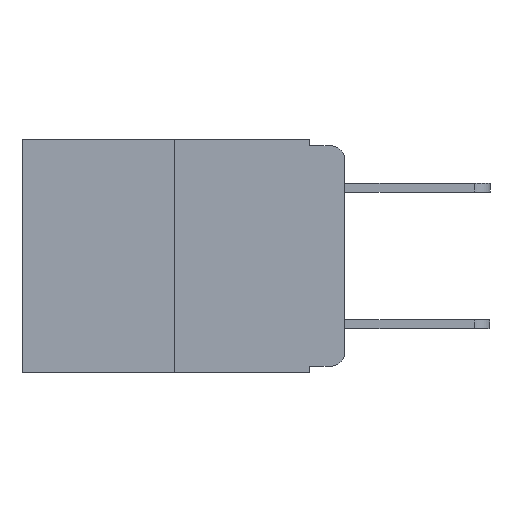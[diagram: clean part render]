
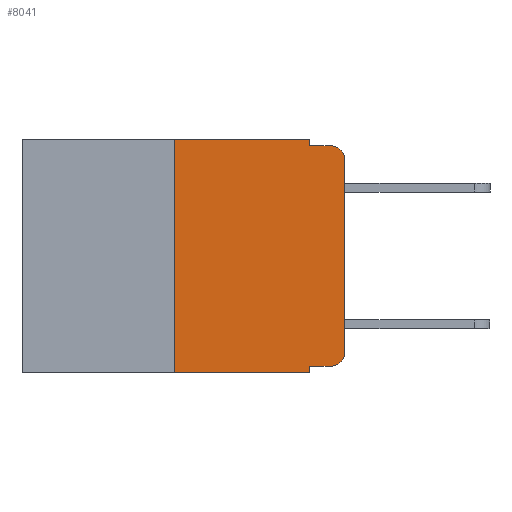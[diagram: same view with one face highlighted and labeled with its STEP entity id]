
A CAD part, left-side view. The second image highlights one B-rep face of the part: STEP entity #8041.
In plain terms, the highlighted planar face has unit normal (-1, 0, 0).
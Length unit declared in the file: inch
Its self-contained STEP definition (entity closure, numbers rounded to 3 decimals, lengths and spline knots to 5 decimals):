
#193 = DIRECTION ( 'NONE',  ( 0., 0., -1. ) ) ;
#194 = EDGE_CURVE ( 'NONE', #2691, #12110, #13412, .T. ) ;
#554 = VECTOR ( 'NONE', #7529, 39.37008 ) ;
#1018 = DIRECTION ( 'NONE',  ( 0., -1., 0. ) ) ;
#1230 = LINE ( 'NONE', #19679, #5658 ) ;
#2228 = CARTESIAN_POINT ( 'NONE',  ( 0., 0.02, -0.313 ) ) ;
#2346 = VECTOR ( 'NONE', #1018, 39.37008 ) ;
#2468 = EDGE_CURVE ( 'NONE', #8242, #2691, #6245, .T. ) ;
#2691 = VERTEX_POINT ( 'NONE', #6325 ) ;
#3019 = CARTESIAN_POINT ( 'NONE',  ( 0., 0.051, 0. ) ) ;
#3304 = DIRECTION ( 'NONE',  ( 0., 0., -1. ) ) ;
#3328 = DIRECTION ( 'NONE',  ( -1., 0., 0. ) ) ;
#3748 = CARTESIAN_POINT ( 'NONE',  ( 0., 0.051, -0.343 ) ) ;
#3849 = CARTESIAN_POINT ( 'NONE',  ( 0., 0.25, 0. ) ) ;
#3960 = EDGE_CURVE ( 'NONE', #19452, #8242, #19490, .T. ) ;
#4040 = VERTEX_POINT ( 'NONE', #14289 ) ;
#4046 = CARTESIAN_POINT ( 'NONE',  ( 0., 0., -0.313 ) ) ;
#4424 = VECTOR ( 'NONE', #7162, 39.37008 ) ;
#4534 = VERTEX_POINT ( 'NONE', #8886 ) ;
#4822 = EDGE_CURVE ( 'NONE', #4040, #15470, #13302, .T. ) ;
#5215 = CARTESIAN_POINT ( 'NONE',  ( 0., 0.02, -0.01 ) ) ;
#5658 = VECTOR ( 'NONE', #9653, 39.37008 ) ;
#6245 = LINE ( 'NONE', #18301, #17659 ) ;
#6325 = CARTESIAN_POINT ( 'NONE',  ( 0., 0., -0.03 ) ) ;
#6693 = CARTESIAN_POINT ( 'NONE',  ( 0., 0.051, -0.333 ) ) ;
#6749 = EDGE_LOOP ( 'NONE', ( #13001, #13119, #13437, #13458, #13741, #13757, #14239, #14386, #14402, #14574 ) ) ;
#7162 = DIRECTION ( 'NONE',  ( 0., 0., 1. ) ) ;
#7529 = DIRECTION ( 'NONE',  ( 0., 0., -1. ) ) ;
#8041 = ADVANCED_FACE ( 'NONE', ( #19569 ), #8360, .F. ) ;
#8242 = VERTEX_POINT ( 'NONE', #4046 ) ;
#8360 = PLANE ( 'NONE',  #9705 ) ;
#8598 = VERTEX_POINT ( 'NONE', #6693 ) ;
#8829 = CARTESIAN_POINT ( 'NONE',  ( 0., 0.25, -0.343 ) ) ;
#8886 = CARTESIAN_POINT ( 'NONE',  ( 0., 0.051, -0.01 ) ) ;
#9170 = LINE ( 'NONE', #3849, #4424 ) ;
#9653 = DIRECTION ( 'NONE',  ( 0., 0., -1. ) ) ;
#9681 = LINE ( 'NONE', #19218, #554 ) ;
#9705 = AXIS2_PLACEMENT_3D ( 'NONE', #11314, #9895, #193 ) ;
#9763 = VECTOR ( 'NONE', #11370, 39.37008 ) ;
#9883 = CARTESIAN_POINT ( 'NONE',  ( 0., 0.051, -0.01 ) ) ;
#9895 = DIRECTION ( 'NONE',  ( 1., 0., 0. ) ) ;
#9986 = LINE ( 'NONE', #17747, #17330 ) ;
#10335 = LINE ( 'NONE', #10609, #2346 ) ;
#10346 = EDGE_CURVE ( 'NONE', #8598, #19452, #10335, .T. ) ;
#10609 = CARTESIAN_POINT ( 'NONE',  ( 0., 0.051, -0.333 ) ) ;
#11038 = CARTESIAN_POINT ( 'NONE',  ( 0., 0.02, -0.333 ) ) ;
#11314 = CARTESIAN_POINT ( 'NONE',  ( 0., 0.473, 0. ) ) ;
#11370 = DIRECTION ( 'NONE',  ( 0., -1., 0. ) ) ;
#11442 = DIRECTION ( 'NONE',  ( -1., 0., 0. ) ) ;
#12110 = VERTEX_POINT ( 'NONE', #5215 ) ;
#13001 = ORIENTED_EDGE ( 'NONE', *, *, #2468, .T. ) ;
#13119 = ORIENTED_EDGE ( 'NONE', *, *, #194, .T. ) ;
#13302 = LINE ( 'NONE', #16129, #16754 ) ;
#13352 = DIRECTION ( 'NONE',  ( 0., 0., 1. ) ) ;
#13412 = CIRCLE ( 'NONE', #14858, 0.02 ) ;
#13437 = ORIENTED_EDGE ( 'NONE', *, *, #19026, .F. ) ;
#13458 = ORIENTED_EDGE ( 'NONE', *, *, #18147, .F. ) ;
#13701 = LINE ( 'NONE', #9883, #9763 ) ;
#13741 = ORIENTED_EDGE ( 'NONE', *, *, #4822, .F. ) ;
#13757 = ORIENTED_EDGE ( 'NONE', *, *, #16285, .F. ) ;
#14239 = ORIENTED_EDGE ( 'NONE', *, *, #19257, .T. ) ;
#14289 = CARTESIAN_POINT ( 'NONE',  ( 0., 0.25, 0. ) ) ;
#14386 = ORIENTED_EDGE ( 'NONE', *, *, #15292, .F. ) ;
#14402 = ORIENTED_EDGE ( 'NONE', *, *, #10346, .T. ) ;
#14574 = ORIENTED_EDGE ( 'NONE', *, *, #3960, .T. ) ;
#14858 = AXIS2_PLACEMENT_3D ( 'NONE', #16600, #11442, #16247 ) ;
#15068 = VERTEX_POINT ( 'NONE', #3748 ) ;
#15163 = VERTEX_POINT ( 'NONE', #8829 ) ;
#15292 = EDGE_CURVE ( 'NONE', #8598, #15068, #9681, .T. ) ;
#15470 = VERTEX_POINT ( 'NONE', #3019 ) ;
#16094 = DIRECTION ( 'NONE',  ( 0., -1., 0. ) ) ;
#16129 = CARTESIAN_POINT ( 'NONE',  ( 0., 0.473, 0. ) ) ;
#16247 = DIRECTION ( 'NONE',  ( 0., 0., -1. ) ) ;
#16285 = EDGE_CURVE ( 'NONE', #15163, #4040, #9170, .T. ) ;
#16600 = CARTESIAN_POINT ( 'NONE',  ( 0., 0.02, -0.03 ) ) ;
#16754 = VECTOR ( 'NONE', #16094, 39.37008 ) ;
#17330 = VECTOR ( 'NONE', #19084, 39.37008 ) ;
#17659 = VECTOR ( 'NONE', #13352, 39.37008 ) ;
#17747 = CARTESIAN_POINT ( 'NONE',  ( 0., 0.473, -0.343 ) ) ;
#18147 = EDGE_CURVE ( 'NONE', #15470, #4534, #1230, .T. ) ;
#18301 = CARTESIAN_POINT ( 'NONE',  ( 0., 0., 0. ) ) ;
#18970 = AXIS2_PLACEMENT_3D ( 'NONE', #2228, #3328, #3304 ) ;
#19026 = EDGE_CURVE ( 'NONE', #4534, #12110, #13701, .T. ) ;
#19084 = DIRECTION ( 'NONE',  ( 0., -1., 0. ) ) ;
#19218 = CARTESIAN_POINT ( 'NONE',  ( 0., 0.051, 0. ) ) ;
#19257 = EDGE_CURVE ( 'NONE', #15163, #15068, #9986, .T. ) ;
#19452 = VERTEX_POINT ( 'NONE', #11038 ) ;
#19490 = CIRCLE ( 'NONE', #18970, 0.02 ) ;
#19569 = FACE_OUTER_BOUND ( 'NONE', #6749, .T. ) ;
#19679 = CARTESIAN_POINT ( 'NONE',  ( 0., 0.051, 0. ) ) ;
